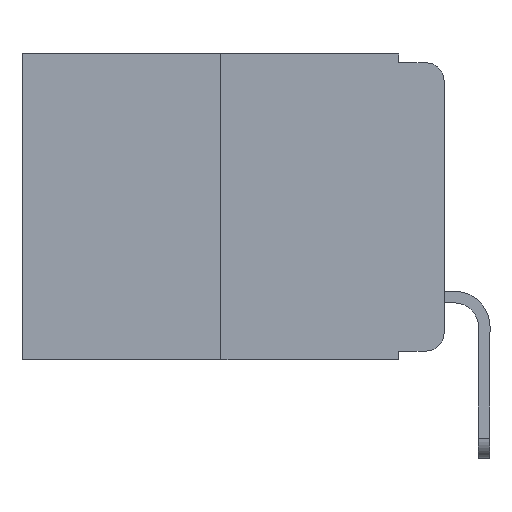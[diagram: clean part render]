
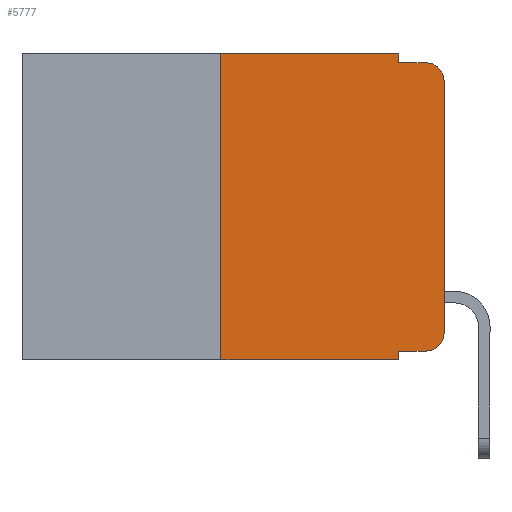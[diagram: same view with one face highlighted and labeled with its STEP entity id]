
A CAD part, left-side view. The second image highlights one B-rep face of the part: STEP entity #5777.
In plain terms, the highlighted planar face has unit normal (-1, 0, 0).
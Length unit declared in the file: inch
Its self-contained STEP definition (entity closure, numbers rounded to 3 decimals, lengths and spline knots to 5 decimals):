
#128 = CARTESIAN_POINT ( 'NONE',  ( 0., 0.473, 0. ) ) ;
#413 = DIRECTION ( 'NONE',  ( 0., -1., 0. ) ) ;
#518 = CARTESIAN_POINT ( 'NONE',  ( 0., 0.051, -0.333 ) ) ;
#595 = LINE ( 'NONE', #1418, #9891 ) ;
#769 = ORIENTED_EDGE ( 'NONE', *, *, #4658, .F. ) ;
#790 = VERTEX_POINT ( 'NONE', #4186 ) ;
#1086 = DIRECTION ( 'NONE',  ( 0., 0., -1. ) ) ;
#1206 = VECTOR ( 'NONE', #3678, 39.37008 ) ;
#1314 = ORIENTED_EDGE ( 'NONE', *, *, #10317, .T. ) ;
#1418 = CARTESIAN_POINT ( 'NONE',  ( 0., 0., 0. ) ) ;
#1525 = DIRECTION ( 'NONE',  ( 1., 0., 0. ) ) ;
#1610 = ORIENTED_EDGE ( 'NONE', *, *, #4582, .F. ) ;
#1868 = FACE_OUTER_BOUND ( 'NONE', #4957, .T. ) ;
#1969 = CARTESIAN_POINT ( 'NONE',  ( 0., 0.051, -0.343 ) ) ;
#2160 = CARTESIAN_POINT ( 'NONE',  ( 0., 0., -0.313 ) ) ;
#2258 = VERTEX_POINT ( 'NONE', #8951 ) ;
#2562 = CARTESIAN_POINT ( 'NONE',  ( 0., 0.473, 0. ) ) ;
#2694 = PLANE ( 'NONE',  #10372 ) ;
#2771 = VERTEX_POINT ( 'NONE', #10924 ) ;
#3288 = ORIENTED_EDGE ( 'NONE', *, *, #3719, .T. ) ;
#3587 = VERTEX_POINT ( 'NONE', #1969 ) ;
#3614 = VERTEX_POINT ( 'NONE', #8236 ) ;
#3678 = DIRECTION ( 'NONE',  ( 0., 0., -1. ) ) ;
#3705 = CIRCLE ( 'NONE', #10727, 0.02 ) ;
#3719 = EDGE_CURVE ( 'NONE', #5367, #3839, #595, .T. ) ;
#3791 = VECTOR ( 'NONE', #1086, 39.37008 ) ;
#3812 = ORIENTED_EDGE ( 'NONE', *, *, #5395, .F. ) ;
#3829 = VERTEX_POINT ( 'NONE', #6591 ) ;
#3839 = VERTEX_POINT ( 'NONE', #9959 ) ;
#3873 = AXIS2_PLACEMENT_3D ( 'NONE', #10261, #10421, #6015 ) ;
#4059 = VECTOR ( 'NONE', #8949, 39.37008 ) ;
#4186 = CARTESIAN_POINT ( 'NONE',  ( 0., 0.02, -0.01 ) ) ;
#4189 = LINE ( 'NONE', #6650, #4469 ) ;
#4285 = ORIENTED_EDGE ( 'NONE', *, *, #4580, .T. ) ;
#4324 = CIRCLE ( 'NONE', #3873, 0.02 ) ;
#4469 = VECTOR ( 'NONE', #4956, 39.37008 ) ;
#4580 = EDGE_CURVE ( 'NONE', #3839, #790, #4324, .T. ) ;
#4582 = EDGE_CURVE ( 'NONE', #2258, #790, #6592, .T. ) ;
#4658 = EDGE_CURVE ( 'NONE', #2771, #2258, #8395, .T. ) ;
#4748 = CARTESIAN_POINT ( 'NONE',  ( 0., 0.051, 0. ) ) ;
#4755 = VERTEX_POINT ( 'NONE', #5901 ) ;
#4901 = EDGE_CURVE ( 'NONE', #4755, #3829, #4189, .T. ) ;
#4956 = DIRECTION ( 'NONE',  ( 0., 0., 1. ) ) ;
#4957 = EDGE_LOOP ( 'NONE', ( #3288, #4285, #1610, #769, #5228, #8744, #1314, #3812, #7501, #11418 ) ) ;
#5217 = LINE ( 'NONE', #9764, #4059 ) ;
#5228 = ORIENTED_EDGE ( 'NONE', *, *, #7378, .F. ) ;
#5367 = VERTEX_POINT ( 'NONE', #2160 ) ;
#5395 = EDGE_CURVE ( 'NONE', #3614, #3587, #8457, .T. ) ;
#5455 = DIRECTION ( 'NONE',  ( 0., -1., 0. ) ) ;
#5537 = EDGE_CURVE ( 'NONE', #3614, #7153, #9075, .T. ) ;
#5649 = EDGE_CURVE ( 'NONE', #7153, #5367, #3705, .T. ) ;
#5777 = ADVANCED_FACE ( 'NONE', ( #1868 ), #2694, .F. ) ;
#5901 = CARTESIAN_POINT ( 'NONE',  ( 0., 0.25, -0.343 ) ) ;
#5959 = VECTOR ( 'NONE', #413, 39.37008 ) ;
#6015 = DIRECTION ( 'NONE',  ( 0., 0., -1. ) ) ;
#6250 = DIRECTION ( 'NONE',  ( 0., 0., 1. ) ) ;
#6387 = DIRECTION ( 'NONE',  ( 0., 0., -1. ) ) ;
#6397 = DIRECTION ( 'NONE',  ( -1., 0., 0. ) ) ;
#6422 = CARTESIAN_POINT ( 'NONE',  ( 0., 0.02, -0.313 ) ) ;
#6591 = CARTESIAN_POINT ( 'NONE',  ( 0., 0.25, 0. ) ) ;
#6592 = LINE ( 'NONE', #10283, #8651 ) ;
#6650 = CARTESIAN_POINT ( 'NONE',  ( 0., 0.25, 0. ) ) ;
#7153 = VERTEX_POINT ( 'NONE', #9228 ) ;
#7194 = CARTESIAN_POINT ( 'NONE',  ( 0., 0.051, 0. ) ) ;
#7204 = DIRECTION ( 'NONE',  ( 0., 0., -1. ) ) ;
#7378 = EDGE_CURVE ( 'NONE', #3829, #2771, #8556, .T. ) ;
#7501 = ORIENTED_EDGE ( 'NONE', *, *, #5537, .T. ) ;
#7599 = DIRECTION ( 'NONE',  ( 0., -1., 0. ) ) ;
#8236 = CARTESIAN_POINT ( 'NONE',  ( 0., 0.051, -0.333 ) ) ;
#8395 = LINE ( 'NONE', #4748, #3791 ) ;
#8457 = LINE ( 'NONE', #7194, #1206 ) ;
#8556 = LINE ( 'NONE', #128, #5959 ) ;
#8651 = VECTOR ( 'NONE', #7599, 39.37008 ) ;
#8744 = ORIENTED_EDGE ( 'NONE', *, *, #4901, .F. ) ;
#8949 = DIRECTION ( 'NONE',  ( 0., -1., 0. ) ) ;
#8951 = CARTESIAN_POINT ( 'NONE',  ( 0., 0.051, -0.01 ) ) ;
#9075 = LINE ( 'NONE', #518, #10987 ) ;
#9228 = CARTESIAN_POINT ( 'NONE',  ( 0., 0.02, -0.333 ) ) ;
#9764 = CARTESIAN_POINT ( 'NONE',  ( 0., 0.473, -0.343 ) ) ;
#9891 = VECTOR ( 'NONE', #6250, 39.37008 ) ;
#9959 = CARTESIAN_POINT ( 'NONE',  ( 0., 0., -0.03 ) ) ;
#10261 = CARTESIAN_POINT ( 'NONE',  ( 0., 0.02, -0.03 ) ) ;
#10283 = CARTESIAN_POINT ( 'NONE',  ( 0., 0.051, -0.01 ) ) ;
#10317 = EDGE_CURVE ( 'NONE', #4755, #3587, #5217, .T. ) ;
#10372 = AXIS2_PLACEMENT_3D ( 'NONE', #2562, #1525, #7204 ) ;
#10421 = DIRECTION ( 'NONE',  ( -1., 0., 0. ) ) ;
#10727 = AXIS2_PLACEMENT_3D ( 'NONE', #6422, #6397, #6387 ) ;
#10924 = CARTESIAN_POINT ( 'NONE',  ( 0., 0.051, 0. ) ) ;
#10987 = VECTOR ( 'NONE', #5455, 39.37008 ) ;
#11418 = ORIENTED_EDGE ( 'NONE', *, *, #5649, .T. ) ;
